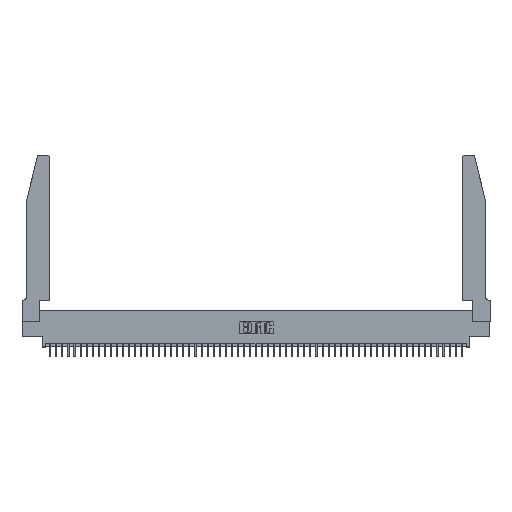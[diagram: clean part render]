
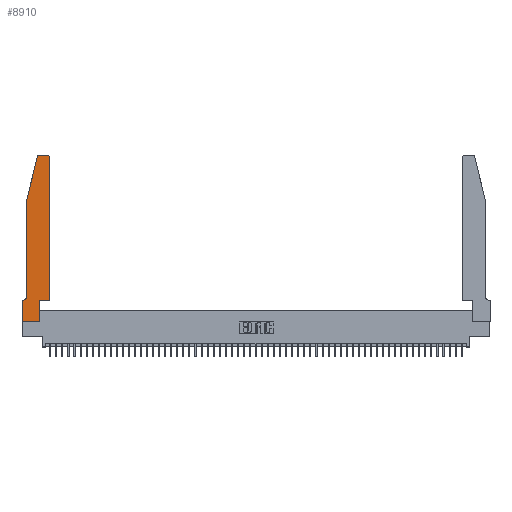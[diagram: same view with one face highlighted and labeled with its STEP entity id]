
A CAD part, top view. The second image highlights one B-rep face of the part: STEP entity #8910.
In plain terms, the highlighted planar face has unit normal (0, 0, 1).
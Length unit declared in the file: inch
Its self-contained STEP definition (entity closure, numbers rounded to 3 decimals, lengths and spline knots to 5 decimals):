
#53 = CARTESIAN_POINT ( 'NONE',  ( 0.0055, 0.35, 0.37 ) ) ;
#243 = CARTESIAN_POINT ( 'NONE',  ( 0.2865, 0.35, 0.37 ) ) ;
#2414 = VECTOR ( 'NONE', #18694, 39.37008 ) ;
#2560 = VERTEX_POINT ( 'NONE', #51878 ) ;
#2577 = LINE ( 'NONE', #41073, #46827 ) ;
#4214 = AXIS2_PLACEMENT_3D ( 'NONE', #50859, #25350, #55105 ) ;
#4364 = VERTEX_POINT ( 'NONE', #5143 ) ;
#4486 = DIRECTION ( 'NONE',  ( -0.239, -0.971, 0. ) ) ;
#4516 = DIRECTION ( 'NONE',  ( 0., 0., 1. ) ) ;
#5092 = VERTEX_POINT ( 'NONE', #48471 ) ;
#5143 = CARTESIAN_POINT ( 'NONE',  ( 0.4505, 0.35, 0.37 ) ) ;
#7642 = ORIENTED_EDGE ( 'NONE', *, *, #16108, .T. ) ;
#8217 = VERTEX_POINT ( 'NONE', #21146 ) ;
#8768 = DIRECTION ( 'NONE',  ( 0., 1., 0. ) ) ;
#8910 = ADVANCED_FACE ( 'NONE', ( #31264 ), #12344, .T. ) ;
#9323 = CARTESIAN_POINT ( 'NONE',  ( 0.4505, 0.35, 0.37 ) ) ;
#9574 = EDGE_LOOP ( 'NONE', ( #25757, #41137, #43756, #7642, #27942, #28703, #25355, #17349, #27488, #28244, #26236, #45726 ) ) ;
#9700 = CIRCLE ( 'NONE', #23343, 0.07 ) ;
#10023 = CARTESIAN_POINT ( 'NONE',  ( 0.0755, 0.35, 0.37 ) ) ;
#10168 = VERTEX_POINT ( 'NONE', #26503 ) ;
#12221 = CARTESIAN_POINT ( 'NONE',  ( 0., 0., 0.37 ) ) ;
#12253 = AXIS2_PLACEMENT_3D ( 'NONE', #50828, #25325, #55077 ) ;
#12344 = PLANE ( 'NONE',  #4214 ) ;
#12931 = EDGE_CURVE ( 'NONE', #8217, #53030, #25506, .T. ) ;
#14277 = VERTEX_POINT ( 'NONE', #17282 ) ;
#16108 = EDGE_CURVE ( 'NONE', #24464, #14277, #28267, .T. ) ;
#16422 = CARTESIAN_POINT ( 'NONE',  ( 0.0055, 0.42, 0.37 ) ) ;
#16896 = VECTOR ( 'NONE', #30170, 39.37008 ) ;
#17282 = CARTESIAN_POINT ( 'NONE',  ( 0.0755, 0.42, 0.37 ) ) ;
#17349 = ORIENTED_EDGE ( 'NONE', *, *, #40250, .T. ) ;
#17407 = EDGE_CURVE ( 'NONE', #53030, #4364, #36844, .T. ) ;
#18694 = DIRECTION ( 'NONE',  ( -1., 0., 0. ) ) ;
#20756 = DIRECTION ( 'NONE',  ( -1., 0., 0. ) ) ;
#21146 = CARTESIAN_POINT ( 'NONE',  ( 0.2865, 0., 0.37 ) ) ;
#21244 = EDGE_CURVE ( 'NONE', #14277, #33903, #9700, .T. ) ;
#21705 = DIRECTION ( 'NONE',  ( 0., 1., 0. ) ) ;
#21879 = CARTESIAN_POINT ( 'NONE',  ( 0.0755, 2., 0.37 ) ) ;
#22022 = CIRCLE ( 'NONE', #12253, 0.03 ) ;
#22807 = VECTOR ( 'NONE', #8768, 39.37008 ) ;
#23343 = AXIS2_PLACEMENT_3D ( 'NONE', #16422, #46326, #20756 ) ;
#24445 = EDGE_CURVE ( 'NONE', #4364, #2560, #33016, .T. ) ;
#24464 = VERTEX_POINT ( 'NONE', #21879 ) ;
#25325 = DIRECTION ( 'NONE',  ( 0., 0., 1. ) ) ;
#25350 = DIRECTION ( 'NONE',  ( 0., 0., 1. ) ) ;
#25355 = ORIENTED_EDGE ( 'NONE', *, *, #51727, .T. ) ;
#25506 = LINE ( 'NONE', #30201, #22807 ) ;
#25757 = ORIENTED_EDGE ( 'NONE', *, *, #30654, .T. ) ;
#26236 = ORIENTED_EDGE ( 'NONE', *, *, #24445, .T. ) ;
#26503 = CARTESIAN_POINT ( 'NONE',  ( 0., 0., 0.37 ) ) ;
#26559 = VECTOR ( 'NONE', #33714, 39.37008 ) ;
#26634 = VERTEX_POINT ( 'NONE', #39397 ) ;
#27402 = LINE ( 'NONE', #30242, #51394 ) ;
#27488 = ORIENTED_EDGE ( 'NONE', *, *, #12931, .T. ) ;
#27561 = CIRCLE ( 'NONE', #41748, 0.03 ) ;
#27914 = LINE ( 'NONE', #12221, #26559 ) ;
#27942 = ORIENTED_EDGE ( 'NONE', *, *, #21244, .T. ) ;
#28244 = ORIENTED_EDGE ( 'NONE', *, *, #17407, .T. ) ;
#28267 = LINE ( 'NONE', #54433, #35651 ) ;
#28319 = LINE ( 'NONE', #34525, #16896 ) ;
#28703 = ORIENTED_EDGE ( 'NONE', *, *, #32769, .T. ) ;
#30170 = DIRECTION ( 'NONE',  ( 0., -1., 0. ) ) ;
#30201 = CARTESIAN_POINT ( 'NONE',  ( 0.2865, 0.35, 0.37 ) ) ;
#30242 = CARTESIAN_POINT ( 'NONE',  ( 0.0755, 2., 0.37 ) ) ;
#30276 = CARTESIAN_POINT ( 'NONE',  ( 0.284, 2.72, 0.37 ) ) ;
#30654 = EDGE_CURVE ( 'NONE', #39669, #51429, #2577, .T. ) ;
#30953 = DIRECTION ( 'NONE',  ( 1., 0., 0. ) ) ;
#31264 = FACE_OUTER_BOUND ( 'NONE', #9574, .T. ) ;
#31444 = EDGE_CURVE ( 'NONE', #2560, #39669, #22022, .T. ) ;
#32373 = DIRECTION ( 'NONE',  ( -1., 0., 0. ) ) ;
#32769 = EDGE_CURVE ( 'NONE', #33903, #5092, #47983, .T. ) ;
#32860 = CARTESIAN_POINT ( 'NONE',  ( 0.284, 2.75, 0.37 ) ) ;
#33016 = LINE ( 'NONE', #51528, #52889 ) ;
#33326 = DIRECTION ( 'NONE',  ( 0., -1., 0. ) ) ;
#33714 = DIRECTION ( 'NONE',  ( 1., 0., 0. ) ) ;
#33903 = VERTEX_POINT ( 'NONE', #53 ) ;
#34525 = CARTESIAN_POINT ( 'NONE',  ( 0., 0., 0.37 ) ) ;
#34626 = DIRECTION ( 'NONE',  ( 1., 0., 0. ) ) ;
#35651 = VECTOR ( 'NONE', #33326, 39.37008 ) ;
#36844 = LINE ( 'NONE', #9323, #49416 ) ;
#38767 = CARTESIAN_POINT ( 'NONE',  ( 0.4205, 2.75, 0.37 ) ) ;
#39397 = CARTESIAN_POINT ( 'NONE',  ( 0.25487, 2.72718, 0.37 ) ) ;
#39669 = VERTEX_POINT ( 'NONE', #38767 ) ;
#40250 = EDGE_CURVE ( 'NONE', #10168, #8217, #27914, .T. ) ;
#41073 = CARTESIAN_POINT ( 'NONE',  ( 0.2605, 2.75, 0.37 ) ) ;
#41137 = ORIENTED_EDGE ( 'NONE', *, *, #44122, .T. ) ;
#41748 = AXIS2_PLACEMENT_3D ( 'NONE', #30276, #4516, #34626 ) ;
#43756 = ORIENTED_EDGE ( 'NONE', *, *, #54484, .T. ) ;
#44122 = EDGE_CURVE ( 'NONE', #51429, #26634, #27561, .T. ) ;
#45726 = ORIENTED_EDGE ( 'NONE', *, *, #31444, .T. ) ;
#46326 = DIRECTION ( 'NONE',  ( 0., 0., -1. ) ) ;
#46827 = VECTOR ( 'NONE', #32373, 39.37008 ) ;
#47983 = LINE ( 'NONE', #10023, #2414 ) ;
#48471 = CARTESIAN_POINT ( 'NONE',  ( 0., 0.35, 0.37 ) ) ;
#49416 = VECTOR ( 'NONE', #30953, 39.37008 ) ;
#50828 = CARTESIAN_POINT ( 'NONE',  ( 0.4205, 2.72, 0.37 ) ) ;
#50859 = CARTESIAN_POINT ( 'NONE',  ( 0., 0.35, 0.37 ) ) ;
#51394 = VECTOR ( 'NONE', #4486, 39.37008 ) ;
#51429 = VERTEX_POINT ( 'NONE', #32860 ) ;
#51528 = CARTESIAN_POINT ( 'NONE',  ( 0.4505, 0.35, 0.37 ) ) ;
#51727 = EDGE_CURVE ( 'NONE', #5092, #10168, #28319, .T. ) ;
#51878 = CARTESIAN_POINT ( 'NONE',  ( 0.4505, 2.72, 0.37 ) ) ;
#52889 = VECTOR ( 'NONE', #21705, 39.37008 ) ;
#53030 = VERTEX_POINT ( 'NONE', #243 ) ;
#54433 = CARTESIAN_POINT ( 'NONE',  ( 0.0755, 2., 0.37 ) ) ;
#54484 = EDGE_CURVE ( 'NONE', #26634, #24464, #27402, .T. ) ;
#55077 = DIRECTION ( 'NONE',  ( 1., 0., 0. ) ) ;
#55105 = DIRECTION ( 'NONE',  ( 1., 0., 0. ) ) ;
